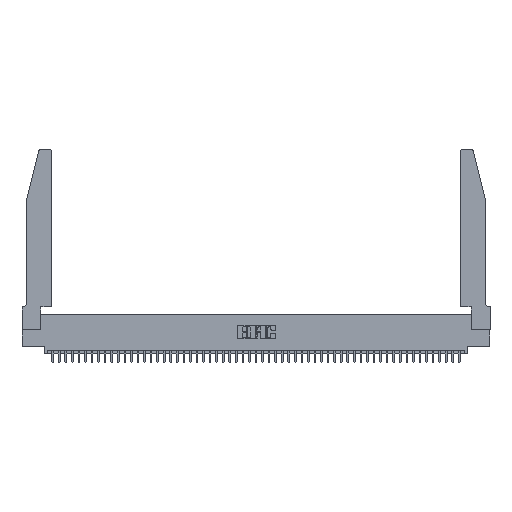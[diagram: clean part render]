
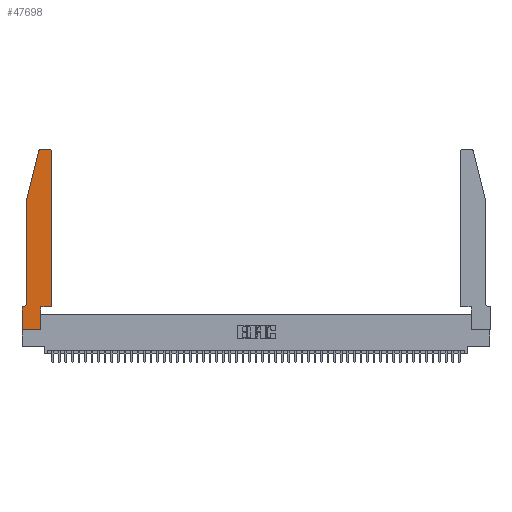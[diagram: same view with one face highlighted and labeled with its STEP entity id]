
A CAD part, top view. The second image highlights one B-rep face of the part: STEP entity #47698.
In plain terms, the highlighted planar face has unit normal (0, 0, 1).
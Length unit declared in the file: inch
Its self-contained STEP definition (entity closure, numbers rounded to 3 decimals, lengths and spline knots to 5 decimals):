
#324 = LINE ( 'NONE', #35272, #32060 ) ;
#412 = ORIENTED_EDGE ( 'NONE', *, *, #34899, .T. ) ;
#744 = VERTEX_POINT ( 'NONE', #38175 ) ;
#812 = ORIENTED_EDGE ( 'NONE', *, *, #23618, .T. ) ;
#1594 = CARTESIAN_POINT ( 'NONE',  ( 0., 0., 0.37 ) ) ;
#2279 = LINE ( 'NONE', #37701, #26494 ) ;
#2891 = CARTESIAN_POINT ( 'NONE',  ( 0.4205, 2.72, 0.37 ) ) ;
#3297 = VERTEX_POINT ( 'NONE', #35032 ) ;
#3607 = ORIENTED_EDGE ( 'NONE', *, *, #13884, .T. ) ;
#4480 = AXIS2_PLACEMENT_3D ( 'NONE', #33099, #36782, #40781 ) ;
#5654 = AXIS2_PLACEMENT_3D ( 'NONE', #33855, #29854, #18191 ) ;
#5972 = ORIENTED_EDGE ( 'NONE', *, *, #19405, .T. ) ;
#7775 = CARTESIAN_POINT ( 'NONE',  ( 0.0055, 0.35, 0.37 ) ) ;
#8416 = EDGE_CURVE ( 'NONE', #40345, #40354, #17221, .T. ) ;
#8518 = ORIENTED_EDGE ( 'NONE', *, *, #9913, .T. ) ;
#9913 = EDGE_CURVE ( 'NONE', #744, #40345, #23533, .T. ) ;
#10171 = CARTESIAN_POINT ( 'NONE',  ( 0.4505, 0.35, 0.37 ) ) ;
#10289 = LINE ( 'NONE', #42620, #41993 ) ;
#11801 = DIRECTION ( 'NONE',  ( -0.239, -0.971, 0. ) ) ;
#12427 = DIRECTION ( 'NONE',  ( -1., 0., 0. ) ) ;
#12850 = CIRCLE ( 'NONE', #15261, 0.03 ) ;
#13369 = VERTEX_POINT ( 'NONE', #25769 ) ;
#13884 = EDGE_CURVE ( 'NONE', #26080, #50314, #26855, .T. ) ;
#14594 = DIRECTION ( 'NONE',  ( -1., 0., 0. ) ) ;
#15215 = DIRECTION ( 'NONE',  ( 1., 0., 0. ) ) ;
#15260 = DIRECTION ( 'NONE',  ( 0., 0., -1. ) ) ;
#15261 = AXIS2_PLACEMENT_3D ( 'NONE', #2891, #38370, #15215 ) ;
#15629 = VECTOR ( 'NONE', #28258, 39.37008 ) ;
#16281 = CARTESIAN_POINT ( 'NONE',  ( 0.284, 2.75, 0.37 ) ) ;
#17221 = CIRCLE ( 'NONE', #5654, 0.03 ) ;
#18166 = EDGE_CURVE ( 'NONE', #20328, #23981, #2279, .T. ) ;
#18191 = DIRECTION ( 'NONE',  ( 1., 0., 0. ) ) ;
#18383 = EDGE_CURVE ( 'NONE', #23870, #744, #12850, .T. ) ;
#19291 = VERTEX_POINT ( 'NONE', #1594 ) ;
#19405 = EDGE_CURVE ( 'NONE', #19291, #20328, #10289, .T. ) ;
#20328 = VERTEX_POINT ( 'NONE', #45076 ) ;
#20546 = EDGE_CURVE ( 'NONE', #13369, #23870, #30038, .T. ) ;
#20720 = AXIS2_PLACEMENT_3D ( 'NONE', #22554, #15260, #14594 ) ;
#21434 = PLANE ( 'NONE',  #4480 ) ;
#22554 = CARTESIAN_POINT ( 'NONE',  ( 0.0055, 0.42, 0.37 ) ) ;
#23533 = LINE ( 'NONE', #34450, #33549 ) ;
#23618 = EDGE_CURVE ( 'NONE', #50314, #45341, #29229, .T. ) ;
#23870 = VERTEX_POINT ( 'NONE', #23904 ) ;
#23904 = CARTESIAN_POINT ( 'NONE',  ( 0.4505, 2.72, 0.37 ) ) ;
#23981 = VERTEX_POINT ( 'NONE', #36301 ) ;
#24258 = CARTESIAN_POINT ( 'NONE',  ( 0.25487, 2.72718, 0.37 ) ) ;
#24924 = EDGE_CURVE ( 'NONE', #23981, #13369, #33537, .T. ) ;
#25105 = ORIENTED_EDGE ( 'NONE', *, *, #24924, .T. ) ;
#25129 = ORIENTED_EDGE ( 'NONE', *, *, #18383, .T. ) ;
#25769 = CARTESIAN_POINT ( 'NONE',  ( 0.4505, 0.35, 0.37 ) ) ;
#26080 = VERTEX_POINT ( 'NONE', #35108 ) ;
#26428 = CARTESIAN_POINT ( 'NONE',  ( 0.0755, 0.42, 0.37 ) ) ;
#26494 = VECTOR ( 'NONE', #30163, 39.37008 ) ;
#26855 = LINE ( 'NONE', #40807, #15629 ) ;
#28155 = LINE ( 'NONE', #48422, #44958 ) ;
#28202 = FACE_OUTER_BOUND ( 'NONE', #32116, .T. ) ;
#28258 = DIRECTION ( 'NONE',  ( 0., -1., 0. ) ) ;
#28644 = ORIENTED_EDGE ( 'NONE', *, *, #40150, .T. ) ;
#29229 = CIRCLE ( 'NONE', #20720, 0.07 ) ;
#29579 = ORIENTED_EDGE ( 'NONE', *, *, #20546, .T. ) ;
#29854 = DIRECTION ( 'NONE',  ( 0., 0., 1. ) ) ;
#30038 = LINE ( 'NONE', #38797, #39401 ) ;
#30069 = DIRECTION ( 'NONE',  ( 0., 1., 0. ) ) ;
#30163 = DIRECTION ( 'NONE',  ( 0., 1., 0. ) ) ;
#30591 = VECTOR ( 'NONE', #34953, 39.37008 ) ;
#30922 = CARTESIAN_POINT ( 'NONE',  ( 0., 0., 0.37 ) ) ;
#31025 = VECTOR ( 'NONE', #51331, 39.37008 ) ;
#32060 = VECTOR ( 'NONE', #11801, 39.37008 ) ;
#32116 = EDGE_LOOP ( 'NONE', ( #8518, #45957, #28644, #3607, #812, #33928, #412, #5972, #48534, #25105, #29579, #25129 ) ) ;
#33099 = CARTESIAN_POINT ( 'NONE',  ( 0., 0.35, 0.37 ) ) ;
#33537 = LINE ( 'NONE', #10171, #31025 ) ;
#33549 = VECTOR ( 'NONE', #34263, 39.37008 ) ;
#33855 = CARTESIAN_POINT ( 'NONE',  ( 0.284, 2.72, 0.37 ) ) ;
#33928 = ORIENTED_EDGE ( 'NONE', *, *, #35684, .T. ) ;
#34263 = DIRECTION ( 'NONE',  ( -1., 0., 0. ) ) ;
#34450 = CARTESIAN_POINT ( 'NONE',  ( 0.2605, 2.75, 0.37 ) ) ;
#34899 = EDGE_CURVE ( 'NONE', #3297, #19291, #46803, .T. ) ;
#34953 = DIRECTION ( 'NONE',  ( 0., -1., 0. ) ) ;
#35032 = CARTESIAN_POINT ( 'NONE',  ( 0., 0.35, 0.37 ) ) ;
#35108 = CARTESIAN_POINT ( 'NONE',  ( 0.0755, 2., 0.37 ) ) ;
#35272 = CARTESIAN_POINT ( 'NONE',  ( 0.0755, 2., 0.37 ) ) ;
#35684 = EDGE_CURVE ( 'NONE', #45341, #3297, #28155, .T. ) ;
#36301 = CARTESIAN_POINT ( 'NONE',  ( 0.2865, 0.35, 0.37 ) ) ;
#36782 = DIRECTION ( 'NONE',  ( 0., 0., 1. ) ) ;
#37701 = CARTESIAN_POINT ( 'NONE',  ( 0.2865, 0.35, 0.37 ) ) ;
#38175 = CARTESIAN_POINT ( 'NONE',  ( 0.4205, 2.75, 0.37 ) ) ;
#38370 = DIRECTION ( 'NONE',  ( 0., 0., 1. ) ) ;
#38797 = CARTESIAN_POINT ( 'NONE',  ( 0.4505, 0.35, 0.37 ) ) ;
#39401 = VECTOR ( 'NONE', #30069, 39.37008 ) ;
#40150 = EDGE_CURVE ( 'NONE', #40354, #26080, #324, .T. ) ;
#40345 = VERTEX_POINT ( 'NONE', #16281 ) ;
#40354 = VERTEX_POINT ( 'NONE', #24258 ) ;
#40781 = DIRECTION ( 'NONE',  ( 1., 0., 0. ) ) ;
#40807 = CARTESIAN_POINT ( 'NONE',  ( 0.0755, 2., 0.37 ) ) ;
#41993 = VECTOR ( 'NONE', #49785, 39.37008 ) ;
#42620 = CARTESIAN_POINT ( 'NONE',  ( 0., 0., 0.37 ) ) ;
#44958 = VECTOR ( 'NONE', #12427, 39.37008 ) ;
#45076 = CARTESIAN_POINT ( 'NONE',  ( 0.2865, 0., 0.37 ) ) ;
#45341 = VERTEX_POINT ( 'NONE', #7775 ) ;
#45957 = ORIENTED_EDGE ( 'NONE', *, *, #8416, .T. ) ;
#46803 = LINE ( 'NONE', #30922, #30591 ) ;
#47698 = ADVANCED_FACE ( 'NONE', ( #28202 ), #21434, .T. ) ;
#48422 = CARTESIAN_POINT ( 'NONE',  ( 0.0755, 0.35, 0.37 ) ) ;
#48534 = ORIENTED_EDGE ( 'NONE', *, *, #18166, .T. ) ;
#49785 = DIRECTION ( 'NONE',  ( 1., 0., 0. ) ) ;
#50314 = VERTEX_POINT ( 'NONE', #26428 ) ;
#51331 = DIRECTION ( 'NONE',  ( 1., 0., 0. ) ) ;
